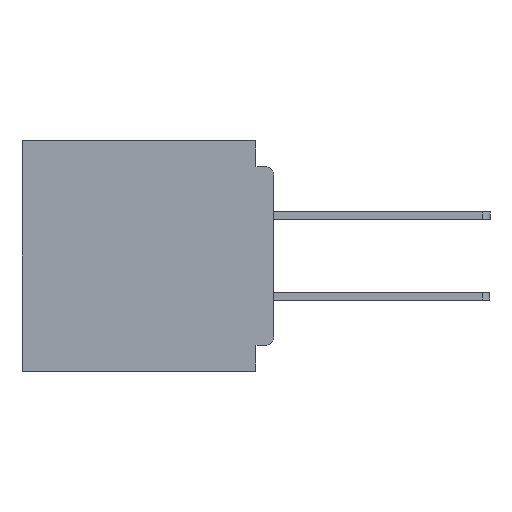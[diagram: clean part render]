
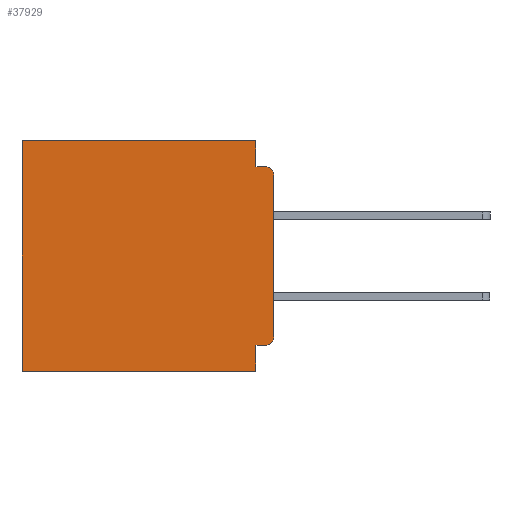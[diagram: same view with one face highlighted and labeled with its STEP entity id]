
A CAD part, left-side view. The second image highlights one B-rep face of the part: STEP entity #37929.
In plain terms, the highlighted planar face has unit normal (-1, 0, 0).
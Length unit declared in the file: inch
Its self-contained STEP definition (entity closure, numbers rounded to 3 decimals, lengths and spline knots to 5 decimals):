
#19 = CARTESIAN_POINT ( 'NONE',  ( 0.3, 0.437, 0. ) ) ;
#571 = CIRCLE ( 'NONE', #38805, 0.015 ) ;
#1421 = DIRECTION ( 'NONE',  ( 0., 1., 0. ) ) ;
#2555 = DIRECTION ( 'NONE',  ( 1., 0., 0. ) ) ;
#2818 = EDGE_CURVE ( 'NONE', #27631, #14311, #36414, .T. ) ;
#3876 = CARTESIAN_POINT ( 'NONE',  ( 0.3, 0.031, -0.355 ) ) ;
#3882 = EDGE_CURVE ( 'NONE', #29953, #44838, #18888, .T. ) ;
#4438 = CARTESIAN_POINT ( 'NONE',  ( 0.3, 0., -0.06 ) ) ;
#4797 = CARTESIAN_POINT ( 'NONE',  ( 0.3, 0., -0.4 ) ) ;
#5026 = EDGE_CURVE ( 'NONE', #14311, #41414, #34551, .T. ) ;
#5433 = CARTESIAN_POINT ( 'NONE',  ( 0.3, 0.031, -0.045 ) ) ;
#7077 = LINE ( 'NONE', #23555, #43944 ) ;
#7115 = DIRECTION ( 'NONE',  ( -1., 0., 0. ) ) ;
#7271 = VECTOR ( 'NONE', #23694, 39.37008 ) ;
#8331 = VECTOR ( 'NONE', #1421, 39.37008 ) ;
#8393 = DIRECTION ( 'NONE',  ( 0., 1., 0. ) ) ;
#9157 = VERTEX_POINT ( 'NONE', #15953 ) ;
#9430 = DIRECTION ( 'NONE',  ( -1., 0., 0. ) ) ;
#14311 = VERTEX_POINT ( 'NONE', #19 ) ;
#15242 = EDGE_CURVE ( 'NONE', #29953, #32995, #26339, .T. ) ;
#15953 = CARTESIAN_POINT ( 'NONE',  ( 0.3, 0.015, -0.045 ) ) ;
#15998 = VECTOR ( 'NONE', #36906, 39.37008 ) ;
#16396 = CARTESIAN_POINT ( 'NONE',  ( 0.3, 0.437, -0.4 ) ) ;
#16507 = EDGE_CURVE ( 'NONE', #44838, #44585, #16671, .T. ) ;
#16671 = LINE ( 'NONE', #37992, #7271 ) ;
#17277 = VECTOR ( 'NONE', #33022, 39.37008 ) ;
#17794 = LINE ( 'NONE', #4797, #35792 ) ;
#18282 = EDGE_CURVE ( 'NONE', #24072, #32995, #7077, .T. ) ;
#18763 = LINE ( 'NONE', #37875, #36733 ) ;
#18879 = VERTEX_POINT ( 'NONE', #5433 ) ;
#18888 = LINE ( 'NONE', #31342, #8331 ) ;
#22171 = AXIS2_PLACEMENT_3D ( 'NONE', #30818, #9430, #34432 ) ;
#23555 = CARTESIAN_POINT ( 'NONE',  ( 0.3, 0., -0.4 ) ) ;
#23694 = DIRECTION ( 'NONE',  ( 0., 0., -1. ) ) ;
#23898 = CARTESIAN_POINT ( 'NONE',  ( 0.3, 0., -0.4 ) ) ;
#24072 = VERTEX_POINT ( 'NONE', #4438 ) ;
#26093 = EDGE_LOOP ( 'NONE', ( #30548, #31307, #31949, #32823, #35273, #36255, #38303, #39059, #41016, #43282 ) ) ;
#26115 = VECTOR ( 'NONE', #45032, 39.37008 ) ;
#26339 = CIRCLE ( 'NONE', #22171, 0.015 ) ;
#27501 = DIRECTION ( 'NONE',  ( 0., 0., -1. ) ) ;
#27631 = VERTEX_POINT ( 'NONE', #28193 ) ;
#27918 = EDGE_CURVE ( 'NONE', #44585, #41414, #17794, .T. ) ;
#28130 = EDGE_CURVE ( 'NONE', #24072, #9157, #571, .T. ) ;
#28193 = CARTESIAN_POINT ( 'NONE',  ( 0.3, 0.031, 0. ) ) ;
#28488 = CARTESIAN_POINT ( 'NONE',  ( 0.3, 0.015, -0.06 ) ) ;
#28551 = AXIS2_PLACEMENT_3D ( 'NONE', #23898, #2555, #27501 ) ;
#29048 = EDGE_CURVE ( 'NONE', #18879, #9157, #35086, .T. ) ;
#29953 = VERTEX_POINT ( 'NONE', #38520 ) ;
#30548 = ORIENTED_EDGE ( 'NONE', *, *, #18282, .F. ) ;
#30818 = CARTESIAN_POINT ( 'NONE',  ( 0.3, 0.015, -0.34 ) ) ;
#31196 = CARTESIAN_POINT ( 'NONE',  ( 0.3, 0.031, -0.4 ) ) ;
#31231 = FACE_OUTER_BOUND ( 'NONE', #26093, .T. ) ;
#31307 = ORIENTED_EDGE ( 'NONE', *, *, #28130, .T. ) ;
#31342 = CARTESIAN_POINT ( 'NONE',  ( 0.3, 0., -0.355 ) ) ;
#31949 = ORIENTED_EDGE ( 'NONE', *, *, #29048, .F. ) ;
#32090 = DIRECTION ( 'NONE',  ( 0., 0., -1. ) ) ;
#32823 = ORIENTED_EDGE ( 'NONE', *, *, #43819, .F. ) ;
#32995 = VERTEX_POINT ( 'NONE', #37916 ) ;
#33022 = DIRECTION ( 'NONE',  ( 0., 1., 0. ) ) ;
#33232 = CARTESIAN_POINT ( 'NONE',  ( 0.3, 0., 0. ) ) ;
#34432 = DIRECTION ( 'NONE',  ( 0., 0., -1. ) ) ;
#34551 = LINE ( 'NONE', #16396, #26115 ) ;
#35086 = LINE ( 'NONE', #40491, #15998 ) ;
#35273 = ORIENTED_EDGE ( 'NONE', *, *, #2818, .T. ) ;
#35792 = VECTOR ( 'NONE', #8393, 39.37008 ) ;
#36255 = ORIENTED_EDGE ( 'NONE', *, *, #5026, .T. ) ;
#36414 = LINE ( 'NONE', #33232, #17277 ) ;
#36733 = VECTOR ( 'NONE', #41441, 39.37008 ) ;
#36906 = DIRECTION ( 'NONE',  ( 0., -1., 0. ) ) ;
#37875 = CARTESIAN_POINT ( 'NONE',  ( 0.3, 0.031, 0. ) ) ;
#37916 = CARTESIAN_POINT ( 'NONE',  ( 0.3, 0., -0.34 ) ) ;
#37929 = ADVANCED_FACE ( 'NONE', ( #31231 ), #41605, .F. ) ;
#37992 = CARTESIAN_POINT ( 'NONE',  ( 0.3, 0.031, -0.4 ) ) ;
#38303 = ORIENTED_EDGE ( 'NONE', *, *, #27918, .F. ) ;
#38520 = CARTESIAN_POINT ( 'NONE',  ( 0.3, 0.015, -0.355 ) ) ;
#38805 = AXIS2_PLACEMENT_3D ( 'NONE', #28488, #7115, #32090 ) ;
#39059 = ORIENTED_EDGE ( 'NONE', *, *, #16507, .F. ) ;
#40491 = CARTESIAN_POINT ( 'NONE',  ( 0.3, 0., -0.045 ) ) ;
#40760 = CARTESIAN_POINT ( 'NONE',  ( 0.3, 0.437, -0.4 ) ) ;
#41016 = ORIENTED_EDGE ( 'NONE', *, *, #3882, .F. ) ;
#41403 = DIRECTION ( 'NONE',  ( 0., 0., -1. ) ) ;
#41414 = VERTEX_POINT ( 'NONE', #40760 ) ;
#41441 = DIRECTION ( 'NONE',  ( 0., 0., -1. ) ) ;
#41605 = PLANE ( 'NONE',  #28551 ) ;
#43282 = ORIENTED_EDGE ( 'NONE', *, *, #15242, .T. ) ;
#43819 = EDGE_CURVE ( 'NONE', #27631, #18879, #18763, .T. ) ;
#43944 = VECTOR ( 'NONE', #41403, 39.37008 ) ;
#44585 = VERTEX_POINT ( 'NONE', #31196 ) ;
#44838 = VERTEX_POINT ( 'NONE', #3876 ) ;
#45032 = DIRECTION ( 'NONE',  ( 0., 0., -1. ) ) ;
